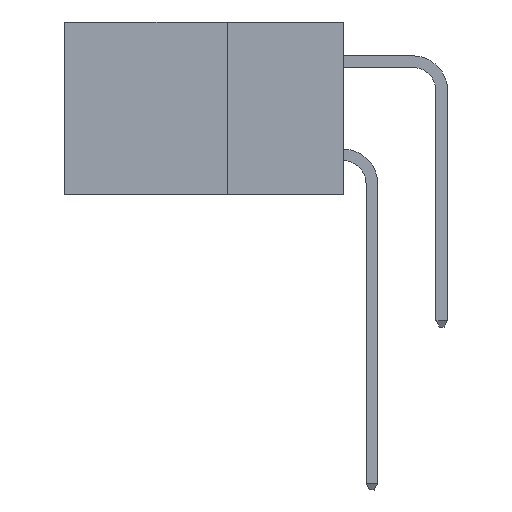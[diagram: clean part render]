
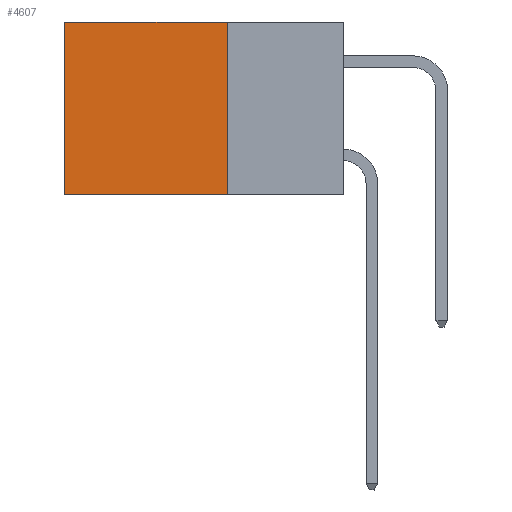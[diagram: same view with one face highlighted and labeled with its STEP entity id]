
A CAD part, left-side view. The second image highlights one B-rep face of the part: STEP entity #4607.
In plain terms, the highlighted planar face has unit normal (-1, 0, 0).
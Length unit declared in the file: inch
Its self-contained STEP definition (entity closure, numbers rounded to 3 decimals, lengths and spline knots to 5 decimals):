
#1399 = ORIENTED_EDGE ( 'NONE', *, *, #5286, .F. ) ;
#1851 = ORIENTED_EDGE ( 'NONE', *, *, #24321, .T. ) ;
#2085 = CARTESIAN_POINT ( 'NONE',  ( 0.298, 0.25, 0. ) ) ;
#2444 = FACE_OUTER_BOUND ( 'NONE', #25174, .T. ) ;
#2792 = CARTESIAN_POINT ( 'NONE',  ( 0.298, 0.6, 0. ) ) ;
#3166 = DIRECTION ( 'NONE',  ( 0., 0., -1. ) ) ;
#3505 = VERTEX_POINT ( 'NONE', #2792 ) ;
#4504 = DIRECTION ( 'NONE',  ( 0., 0., -1. ) ) ;
#4607 = ADVANCED_FACE ( 'NONE', ( #2444 ), #7415, .F. ) ;
#5239 = CARTESIAN_POINT ( 'NONE',  ( 0.298, 0.25, 0. ) ) ;
#5286 = EDGE_CURVE ( 'NONE', #23953, #10326, #22261, .T. ) ;
#5368 = CARTESIAN_POINT ( 'NONE',  ( 0.298, 0.6, -0.37 ) ) ;
#5823 = CARTESIAN_POINT ( 'NONE',  ( 0.298, 0.25, 0. ) ) ;
#6852 = VECTOR ( 'NONE', #19833, 39.37008 ) ;
#7415 = PLANE ( 'NONE',  #18433 ) ;
#8103 = LINE ( 'NONE', #14281, #12628 ) ;
#8495 = CARTESIAN_POINT ( 'NONE',  ( 0.298, 0.25, 0. ) ) ;
#10326 = VERTEX_POINT ( 'NONE', #5368 ) ;
#11271 = ORIENTED_EDGE ( 'NONE', *, *, #13306, .T. ) ;
#12628 = VECTOR ( 'NONE', #4504, 39.37008 ) ;
#13306 = EDGE_CURVE ( 'NONE', #3505, #10326, #8103, .T. ) ;
#13385 = LINE ( 'NONE', #5239, #23033 ) ;
#13806 = LINE ( 'NONE', #8495, #21636 ) ;
#13907 = VERTEX_POINT ( 'NONE', #2085 ) ;
#14281 = CARTESIAN_POINT ( 'NONE',  ( 0.298, 0.6, 0. ) ) ;
#15014 = DIRECTION ( 'NONE',  ( 1., 0., 0. ) ) ;
#17313 = EDGE_CURVE ( 'NONE', #13907, #23953, #13385, .T. ) ;
#18433 = AXIS2_PLACEMENT_3D ( 'NONE', #5823, #15014, #3166 ) ;
#19750 = CARTESIAN_POINT ( 'NONE',  ( 0.298, 0.25, -0.37 ) ) ;
#19833 = DIRECTION ( 'NONE',  ( 0., 1., 0. ) ) ;
#20113 = DIRECTION ( 'NONE',  ( 0., 1., 0. ) ) ;
#20881 = CARTESIAN_POINT ( 'NONE',  ( 0.298, 0.25, -0.37 ) ) ;
#21636 = VECTOR ( 'NONE', #20113, 39.37008 ) ;
#22261 = LINE ( 'NONE', #19750, #6852 ) ;
#23033 = VECTOR ( 'NONE', #24693, 39.37008 ) ;
#23953 = VERTEX_POINT ( 'NONE', #20881 ) ;
#24141 = ORIENTED_EDGE ( 'NONE', *, *, #17313, .F. ) ;
#24321 = EDGE_CURVE ( 'NONE', #13907, #3505, #13806, .T. ) ;
#24693 = DIRECTION ( 'NONE',  ( 0., 0., -1. ) ) ;
#25174 = EDGE_LOOP ( 'NONE', ( #11271, #1399, #24141, #1851 ) ) ;
